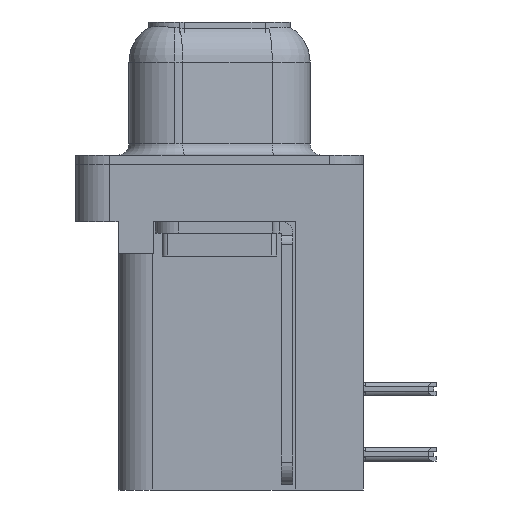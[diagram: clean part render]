
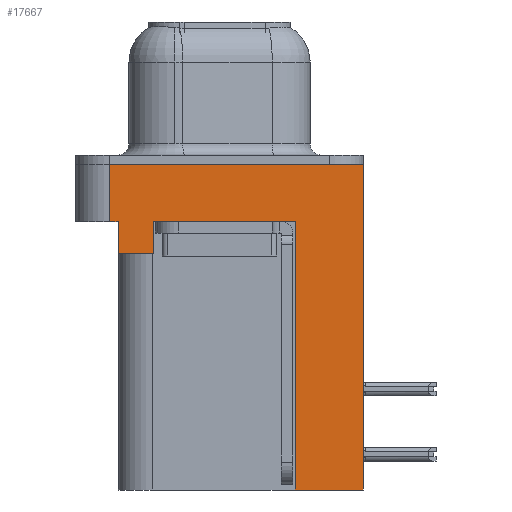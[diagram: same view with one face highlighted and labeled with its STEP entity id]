
A CAD part, left-side view. The second image highlights one B-rep face of the part: STEP entity #17667.
In plain terms, the highlighted planar face has unit normal (-1, 0, 0).
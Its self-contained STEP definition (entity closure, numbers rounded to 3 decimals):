
#364 = CARTESIAN_POINT ( 'NONE',  ( -2.91, -6.275, -2.5 ) ) ;
#1650 = DIRECTION ( 'NONE',  ( 0., 0., 1. ) ) ;
#1682 = LINE ( 'NONE', #4264, #16767 ) ;
#1855 = DIRECTION ( 'NONE',  ( 0., -1., 0. ) ) ;
#3024 = AXIS2_PLACEMENT_3D ( 'NONE', #364, #3279, #32195 ) ;
#3114 = FACE_OUTER_BOUND ( 'NONE', #32063, .T. ) ;
#3200 = LINE ( 'NONE', #11295, #13507 ) ;
#3279 = DIRECTION ( 'NONE',  ( -1., 0., 0. ) ) ;
#3740 = VERTEX_POINT ( 'NONE', #9766 ) ;
#3920 = DIRECTION ( 'NONE',  ( 0., 0., 1. ) ) ;
#4264 = CARTESIAN_POINT ( 'NONE',  ( -2.91, -6.275, -2.5 ) ) ;
#4556 = CARTESIAN_POINT ( 'NONE',  ( -2.91, -6.275, 0. ) ) ;
#4879 = ORIENTED_EDGE ( 'NONE', *, *, #14735, .F. ) ;
#6737 = VECTOR ( 'NONE', #3920, 1000. ) ;
#6956 = VERTEX_POINT ( 'NONE', #4556 ) ;
#7018 = CARTESIAN_POINT ( 'NONE',  ( -2.91, 4.775, -2.5 ) ) ;
#7122 = ORIENTED_EDGE ( 'NONE', *, *, #25682, .T. ) ;
#7494 = LINE ( 'NONE', #10074, #21761 ) ;
#8238 = VERTEX_POINT ( 'NONE', #31447 ) ;
#8502 = CARTESIAN_POINT ( 'NONE',  ( -2.91, 4.775, -2.5 ) ) ;
#8941 = LINE ( 'NONE', #22560, #14910 ) ;
#9036 = VERTEX_POINT ( 'NONE', #21948 ) ;
#9042 = ORIENTED_EDGE ( 'NONE', *, *, #13017, .F. ) ;
#9093 = ORIENTED_EDGE ( 'NONE', *, *, #11973, .F. ) ;
#9532 = ORIENTED_EDGE ( 'NONE', *, *, #28751, .T. ) ;
#9766 = CARTESIAN_POINT ( 'NONE',  ( -2.91, 4.775, 0. ) ) ;
#9771 = CARTESIAN_POINT ( 'NONE',  ( -2.91, -6.275, 0. ) ) ;
#10074 = CARTESIAN_POINT ( 'NONE',  ( -2.91, -3.295, -14.2 ) ) ;
#10720 = ORIENTED_EDGE ( 'NONE', *, *, #13413, .T. ) ;
#10934 = LINE ( 'NONE', #8502, #12668 ) ;
#11295 = CARTESIAN_POINT ( 'NONE',  ( -2.91, -6.275, -2.5 ) ) ;
#11577 = CARTESIAN_POINT ( 'NONE',  ( -2.91, 2.895, -2.5 ) ) ;
#11689 = ORIENTED_EDGE ( 'NONE', *, *, #29489, .F. ) ;
#11838 = LINE ( 'NONE', #22356, #30877 ) ;
#11973 = EDGE_CURVE ( 'NONE', #27654, #3740, #10934, .T. ) ;
#12668 = VECTOR ( 'NONE', #13684, 1000. ) ;
#13017 = EDGE_CURVE ( 'NONE', #9036, #27227, #8941, .T. ) ;
#13284 = CARTESIAN_POINT ( 'NONE',  ( -2.91, 4.425, -3.9 ) ) ;
#13413 = EDGE_CURVE ( 'NONE', #20728, #6956, #11838, .T. ) ;
#13507 = VECTOR ( 'NONE', #24371, 1000. ) ;
#13684 = DIRECTION ( 'NONE',  ( 0., 0., 1. ) ) ;
#13777 = PLANE ( 'NONE',  #3024 ) ;
#13874 = CARTESIAN_POINT ( 'NONE',  ( -2.91, 4.425, -2.5 ) ) ;
#14480 = CARTESIAN_POINT ( 'NONE',  ( -2.91, -3.295, -14.2 ) ) ;
#14657 = EDGE_CURVE ( 'NONE', #8238, #23786, #25272, .T. ) ;
#14735 = EDGE_CURVE ( 'NONE', #3740, #6956, #15447, .T. ) ;
#14910 = VECTOR ( 'NONE', #19440, 1000. ) ;
#15447 = LINE ( 'NONE', #9771, #22711 ) ;
#16767 = VECTOR ( 'NONE', #29906, 1000. ) ;
#17667 = ADVANCED_FACE ( 'NONE', ( #3114 ), #13777, .T. ) ;
#18665 = VECTOR ( 'NONE', #31511, 1000. ) ;
#19440 = DIRECTION ( 'NONE',  ( 0., 0., 1. ) ) ;
#19599 = VECTOR ( 'NONE', #28455, 1000. ) ;
#19769 = EDGE_CURVE ( 'NONE', #30999, #22810, #7494, .T. ) ;
#20728 = VERTEX_POINT ( 'NONE', #31958 ) ;
#21761 = VECTOR ( 'NONE', #1650, 1000. ) ;
#21948 = CARTESIAN_POINT ( 'NONE',  ( -2.91, 4.425, -3.9 ) ) ;
#22356 = CARTESIAN_POINT ( 'NONE',  ( -2.91, -6.275, -2.5 ) ) ;
#22560 = CARTESIAN_POINT ( 'NONE',  ( -2.91, 4.425, -3.9 ) ) ;
#22711 = VECTOR ( 'NONE', #1855, 1000. ) ;
#22810 = VERTEX_POINT ( 'NONE', #24100 ) ;
#23456 = LINE ( 'NONE', #13284, #19599 ) ;
#23786 = VERTEX_POINT ( 'NONE', #11577 ) ;
#24100 = CARTESIAN_POINT ( 'NONE',  ( -2.91, -3.295, -2.5 ) ) ;
#24371 = DIRECTION ( 'NONE',  ( 0., -1., 0. ) ) ;
#25272 = LINE ( 'NONE', #33186, #6737 ) ;
#25682 = EDGE_CURVE ( 'NONE', #27654, #27227, #1682, .T. ) ;
#26362 = LINE ( 'NONE', #29598, #18665 ) ;
#26946 = ORIENTED_EDGE ( 'NONE', *, *, #19769, .F. ) ;
#27227 = VERTEX_POINT ( 'NONE', #13874 ) ;
#27654 = VERTEX_POINT ( 'NONE', #7018 ) ;
#28070 = ORIENTED_EDGE ( 'NONE', *, *, #14657, .T. ) ;
#28455 = DIRECTION ( 'NONE',  ( 0., 1., 0. ) ) ;
#28751 = EDGE_CURVE ( 'NONE', #23786, #22810, #3200, .T. ) ;
#29489 = EDGE_CURVE ( 'NONE', #8238, #9036, #23456, .T. ) ;
#29598 = CARTESIAN_POINT ( 'NONE',  ( -2.91, -3.295, -14.2 ) ) ;
#29906 = DIRECTION ( 'NONE',  ( 0., -1., 0. ) ) ;
#30877 = VECTOR ( 'NONE', #32845, 1000. ) ;
#30999 = VERTEX_POINT ( 'NONE', #14480 ) ;
#31447 = CARTESIAN_POINT ( 'NONE',  ( -2.91, 2.895, -3.9 ) ) ;
#31511 = DIRECTION ( 'NONE',  ( 0., 1., 0. ) ) ;
#31958 = CARTESIAN_POINT ( 'NONE',  ( -2.91, -6.275, -14.2 ) ) ;
#32063 = EDGE_LOOP ( 'NONE', ( #4879, #9093, #7122, #9042, #11689, #28070, #9532, #26946, #32612, #10720 ) ) ;
#32195 = DIRECTION ( 'NONE',  ( 0., 0., 1. ) ) ;
#32612 = ORIENTED_EDGE ( 'NONE', *, *, #33627, .F. ) ;
#32845 = DIRECTION ( 'NONE',  ( 0., 0., 1. ) ) ;
#33186 = CARTESIAN_POINT ( 'NONE',  ( -2.91, 2.895, -3.9 ) ) ;
#33627 = EDGE_CURVE ( 'NONE', #20728, #30999, #26362, .T. ) ;
